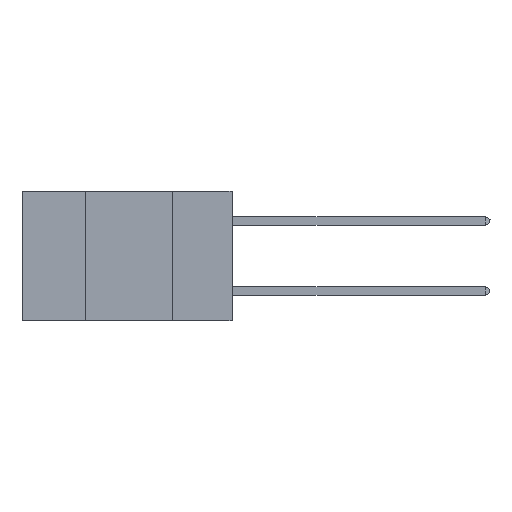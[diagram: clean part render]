
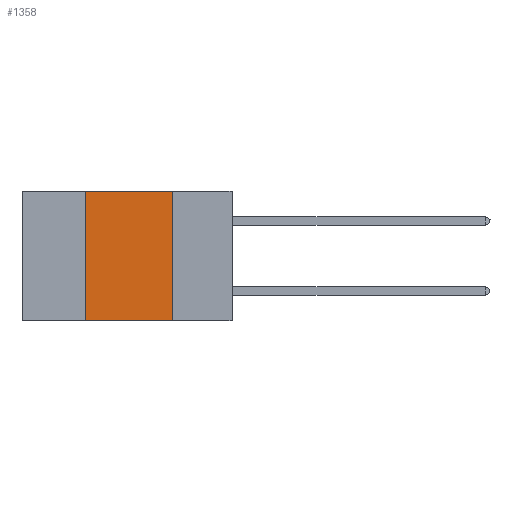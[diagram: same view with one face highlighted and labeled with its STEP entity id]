
A CAD part, left-side view. The second image highlights one B-rep face of the part: STEP entity #1358.
In plain terms, the highlighted planar face has unit normal (-1, 0, 0).
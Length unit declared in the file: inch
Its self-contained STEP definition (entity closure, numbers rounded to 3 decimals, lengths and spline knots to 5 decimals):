
#1330 = CARTESIAN_POINT ( 'NONE',  ( 0., 0.17, 0. ) ) ;
#1358 = ADVANCED_FACE ( 'NONE', ( #18749 ), #11026, .F. ) ;
#1523 = EDGE_LOOP ( 'NONE', ( #10048, #22677, #7051, #3520 ) ) ;
#3509 = CARTESIAN_POINT ( 'NONE',  ( 0., 0.42, 0. ) ) ;
#3520 = ORIENTED_EDGE ( 'NONE', *, *, #23802, .T. ) ;
#4448 = LINE ( 'NONE', #24984, #12089 ) ;
#4956 = CARTESIAN_POINT ( 'NONE',  ( 0., 0.42, -0.37 ) ) ;
#4987 = VERTEX_POINT ( 'NONE', #4956 ) ;
#5850 = VECTOR ( 'NONE', #25001, 39.37008 ) ;
#7051 = ORIENTED_EDGE ( 'NONE', *, *, #11202, .F. ) ;
#7759 = DIRECTION ( 'NONE',  ( 0., 0., 1. ) ) ;
#8183 = CARTESIAN_POINT ( 'NONE',  ( 0., 0.42, 0. ) ) ;
#8867 = CARTESIAN_POINT ( 'NONE',  ( 0., 0.17, 0. ) ) ;
#9819 = LINE ( 'NONE', #8867, #14641 ) ;
#10046 = VECTOR ( 'NONE', #7759, 39.37008 ) ;
#10048 = ORIENTED_EDGE ( 'NONE', *, *, #26222, .F. ) ;
#10646 = CARTESIAN_POINT ( 'NONE',  ( 0., 0.6, -0.37 ) ) ;
#10767 = AXIS2_PLACEMENT_3D ( 'NONE', #23324, #23694, #15528 ) ;
#11026 = PLANE ( 'NONE',  #10767 ) ;
#11202 = EDGE_CURVE ( 'NONE', #4987, #12806, #12278, .T. ) ;
#12032 = CARTESIAN_POINT ( 'NONE',  ( 0., 0.17, -0.37 ) ) ;
#12089 = VECTOR ( 'NONE', #24811, 39.37008 ) ;
#12278 = LINE ( 'NONE', #3509, #10046 ) ;
#12806 = VERTEX_POINT ( 'NONE', #8183 ) ;
#14248 = VERTEX_POINT ( 'NONE', #1330 ) ;
#14641 = VECTOR ( 'NONE', #17062, 39.37008 ) ;
#15528 = DIRECTION ( 'NONE',  ( 0., 0., -1. ) ) ;
#16758 = LINE ( 'NONE', #10646, #5850 ) ;
#17062 = DIRECTION ( 'NONE',  ( 0., 0., -1. ) ) ;
#17232 = EDGE_CURVE ( 'NONE', #12806, #14248, #4448, .T. ) ;
#17584 = VERTEX_POINT ( 'NONE', #12032 ) ;
#18749 = FACE_OUTER_BOUND ( 'NONE', #1523, .T. ) ;
#22677 = ORIENTED_EDGE ( 'NONE', *, *, #17232, .F. ) ;
#23324 = CARTESIAN_POINT ( 'NONE',  ( 0., 0.6, 0. ) ) ;
#23694 = DIRECTION ( 'NONE',  ( 1., 0., 0. ) ) ;
#23802 = EDGE_CURVE ( 'NONE', #4987, #17584, #16758, .T. ) ;
#24811 = DIRECTION ( 'NONE',  ( 0., -1., 0. ) ) ;
#24984 = CARTESIAN_POINT ( 'NONE',  ( 0., 0.6, 0. ) ) ;
#25001 = DIRECTION ( 'NONE',  ( 0., -1., 0. ) ) ;
#26222 = EDGE_CURVE ( 'NONE', #14248, #17584, #9819, .T. ) ;
